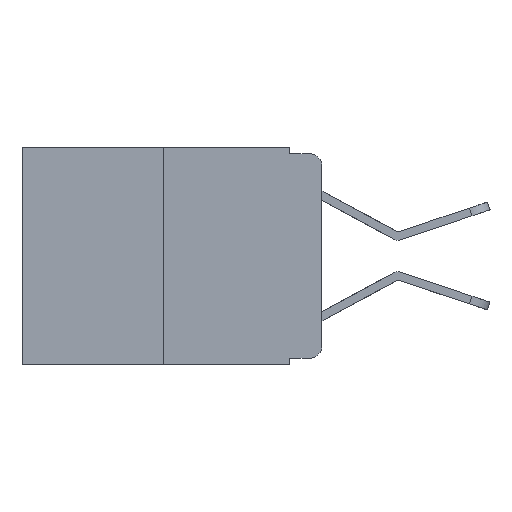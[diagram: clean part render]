
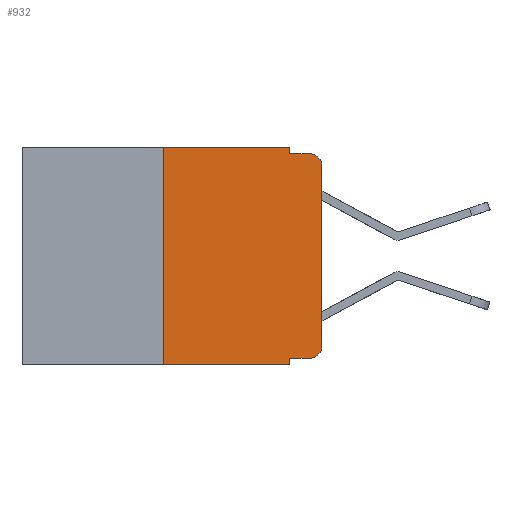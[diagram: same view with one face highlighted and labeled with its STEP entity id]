
A CAD part, left-side view. The second image highlights one B-rep face of the part: STEP entity #932.
In plain terms, the highlighted planar face has unit normal (-1, 0, 0).
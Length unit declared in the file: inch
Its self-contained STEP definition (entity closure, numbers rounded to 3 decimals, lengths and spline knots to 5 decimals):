
#762 = VERTEX_POINT ( 'NONE', #25505 ) ;
#795 = CARTESIAN_POINT ( 'NONE',  ( 0., 0.02, -0.313 ) ) ;
#932 = ADVANCED_FACE ( 'NONE', ( #24701 ), #6821, .F. ) ;
#988 = LINE ( 'NONE', #25416, #10946 ) ;
#2018 = CIRCLE ( 'NONE', #2948, 0.02 ) ;
#2509 = CARTESIAN_POINT ( 'NONE',  ( 0., 0.02, -0.333 ) ) ;
#2524 = EDGE_CURVE ( 'NONE', #3427, #10258, #13478, .T. ) ;
#2860 = DIRECTION ( 'NONE',  ( 0., 0., -1. ) ) ;
#2948 = AXIS2_PLACEMENT_3D ( 'NONE', #795, #14717, #2860 ) ;
#3035 = ORIENTED_EDGE ( 'NONE', *, *, #11989, .T. ) ;
#3342 = ORIENTED_EDGE ( 'NONE', *, *, #3860, .F. ) ;
#3427 = VERTEX_POINT ( 'NONE', #15018 ) ;
#3774 = DIRECTION ( 'NONE',  ( 0., -1., 0. ) ) ;
#3836 = VECTOR ( 'NONE', #19683, 39.37008 ) ;
#3860 = EDGE_CURVE ( 'NONE', #10559, #762, #14978, .T. ) ;
#4042 = VECTOR ( 'NONE', #22250, 39.37008 ) ;
#4709 = VECTOR ( 'NONE', #12907, 39.37008 ) ;
#4772 = VECTOR ( 'NONE', #3774, 39.37008 ) ;
#5610 = CARTESIAN_POINT ( 'NONE',  ( 0., 0.473, -0.343 ) ) ;
#5804 = DIRECTION ( 'NONE',  ( 0., 0., -1. ) ) ;
#6003 = VECTOR ( 'NONE', #12351, 39.37008 ) ;
#6098 = CARTESIAN_POINT ( 'NONE',  ( 0., 0.25, 0. ) ) ;
#6503 = LINE ( 'NONE', #17232, #21649 ) ;
#6679 = DIRECTION ( 'NONE',  ( 1., 0., 0. ) ) ;
#6707 = DIRECTION ( 'NONE',  ( 0., 0., -1. ) ) ;
#6730 = CARTESIAN_POINT ( 'NONE',  ( 0., 0.473, 0. ) ) ;
#6821 = PLANE ( 'NONE',  #18638 ) ;
#7111 = CARTESIAN_POINT ( 'NONE',  ( 0., 0.051, 0. ) ) ;
#7825 = EDGE_CURVE ( 'NONE', #762, #17463, #6503, .T. ) ;
#8182 = VECTOR ( 'NONE', #11138, 39.37008 ) ;
#8285 = ORIENTED_EDGE ( 'NONE', *, *, #2524, .F. ) ;
#8303 = ORIENTED_EDGE ( 'NONE', *, *, #10981, .T. ) ;
#8827 = DIRECTION ( 'NONE',  ( -1., 0., 0. ) ) ;
#9083 = CARTESIAN_POINT ( 'NONE',  ( 0., 0.051, 0. ) ) ;
#10145 = ORIENTED_EDGE ( 'NONE', *, *, #7825, .F. ) ;
#10258 = VERTEX_POINT ( 'NONE', #6098 ) ;
#10476 = EDGE_CURVE ( 'NONE', #20004, #17463, #23347, .T. ) ;
#10559 = VERTEX_POINT ( 'NONE', #7111 ) ;
#10946 = VECTOR ( 'NONE', #5804, 39.37008 ) ;
#10981 = EDGE_CURVE ( 'NONE', #19754, #24077, #2018, .T. ) ;
#11138 = DIRECTION ( 'NONE',  ( 0., 0., 1. ) ) ;
#11989 = EDGE_CURVE ( 'NONE', #3427, #15246, #19895, .T. ) ;
#12351 = DIRECTION ( 'NONE',  ( 0., -1., 0. ) ) ;
#12907 = DIRECTION ( 'NONE',  ( 0., 0., 1. ) ) ;
#12927 = ORIENTED_EDGE ( 'NONE', *, *, #10476, .T. ) ;
#13034 = AXIS2_PLACEMENT_3D ( 'NONE', #20665, #8827, #22640 ) ;
#13478 = LINE ( 'NONE', #25034, #8182 ) ;
#13630 = CARTESIAN_POINT ( 'NONE',  ( 0., 0.02, -0.01 ) ) ;
#13961 = LINE ( 'NONE', #20267, #4042 ) ;
#14457 = EDGE_CURVE ( 'NONE', #24077, #20004, #15222, .T. ) ;
#14717 = DIRECTION ( 'NONE',  ( -1., 0., 0. ) ) ;
#14963 = EDGE_CURVE ( 'NONE', #23420, #19754, #13961, .T. ) ;
#14978 = LINE ( 'NONE', #9083, #3836 ) ;
#15018 = CARTESIAN_POINT ( 'NONE',  ( 0., 0.25, -0.343 ) ) ;
#15222 = LINE ( 'NONE', #24665, #4709 ) ;
#15246 = VERTEX_POINT ( 'NONE', #24961 ) ;
#16601 = CARTESIAN_POINT ( 'NONE',  ( 0., 0.051, -0.333 ) ) ;
#17119 = LINE ( 'NONE', #20187, #6003 ) ;
#17232 = CARTESIAN_POINT ( 'NONE',  ( 0., 0.051, -0.01 ) ) ;
#17463 = VERTEX_POINT ( 'NONE', #13630 ) ;
#18638 = AXIS2_PLACEMENT_3D ( 'NONE', #6730, #6679, #6707 ) ;
#19683 = DIRECTION ( 'NONE',  ( 0., 0., -1. ) ) ;
#19696 = ORIENTED_EDGE ( 'NONE', *, *, #14457, .T. ) ;
#19754 = VERTEX_POINT ( 'NONE', #2509 ) ;
#19895 = LINE ( 'NONE', #5610, #4772 ) ;
#20004 = VERTEX_POINT ( 'NONE', #20861 ) ;
#20187 = CARTESIAN_POINT ( 'NONE',  ( 0., 0.473, 0. ) ) ;
#20267 = CARTESIAN_POINT ( 'NONE',  ( 0., 0.051, -0.333 ) ) ;
#20665 = CARTESIAN_POINT ( 'NONE',  ( 0., 0.02, -0.03 ) ) ;
#20811 = CARTESIAN_POINT ( 'NONE',  ( 0., 0., -0.313 ) ) ;
#20861 = CARTESIAN_POINT ( 'NONE',  ( 0., 0., -0.03 ) ) ;
#21367 = EDGE_LOOP ( 'NONE', ( #19696, #12927, #10145, #3342, #24906, #8285, #3035, #22482, #22182, #8303 ) ) ;
#21566 = EDGE_CURVE ( 'NONE', #23420, #15246, #988, .T. ) ;
#21649 = VECTOR ( 'NONE', #23161, 39.37008 ) ;
#21773 = EDGE_CURVE ( 'NONE', #10258, #10559, #17119, .T. ) ;
#22182 = ORIENTED_EDGE ( 'NONE', *, *, #14963, .T. ) ;
#22250 = DIRECTION ( 'NONE',  ( 0., -1., 0. ) ) ;
#22482 = ORIENTED_EDGE ( 'NONE', *, *, #21566, .F. ) ;
#22640 = DIRECTION ( 'NONE',  ( 0., 0., -1. ) ) ;
#23161 = DIRECTION ( 'NONE',  ( 0., -1., 0. ) ) ;
#23347 = CIRCLE ( 'NONE', #13034, 0.02 ) ;
#23420 = VERTEX_POINT ( 'NONE', #16601 ) ;
#24077 = VERTEX_POINT ( 'NONE', #20811 ) ;
#24665 = CARTESIAN_POINT ( 'NONE',  ( 0., 0., 0. ) ) ;
#24701 = FACE_OUTER_BOUND ( 'NONE', #21367, .T. ) ;
#24906 = ORIENTED_EDGE ( 'NONE', *, *, #21773, .F. ) ;
#24961 = CARTESIAN_POINT ( 'NONE',  ( 0., 0.051, -0.343 ) ) ;
#25034 = CARTESIAN_POINT ( 'NONE',  ( 0., 0.25, 0. ) ) ;
#25416 = CARTESIAN_POINT ( 'NONE',  ( 0., 0.051, 0. ) ) ;
#25505 = CARTESIAN_POINT ( 'NONE',  ( 0., 0.051, -0.01 ) ) ;
